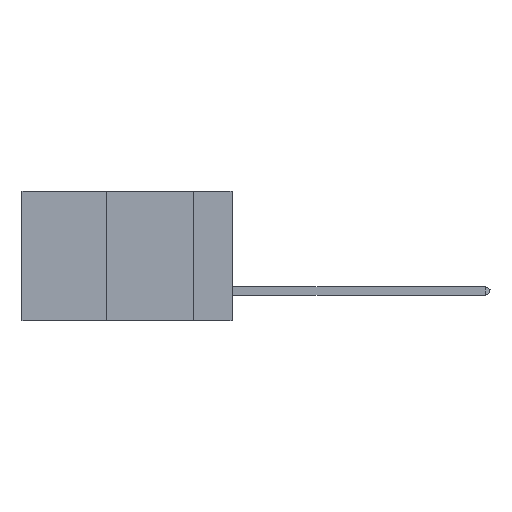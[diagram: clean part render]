
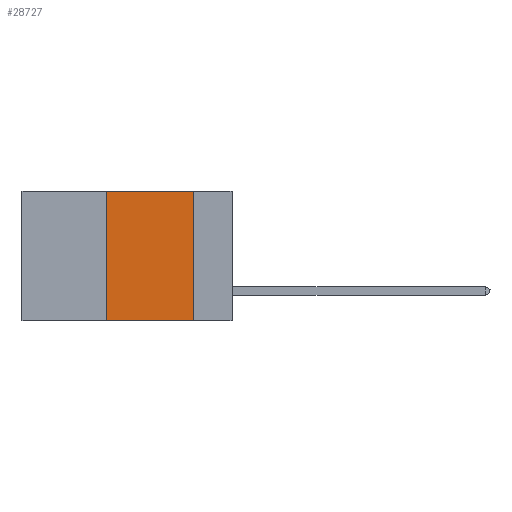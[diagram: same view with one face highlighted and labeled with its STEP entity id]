
A CAD part, left-side view. The second image highlights one B-rep face of the part: STEP entity #28727.
In plain terms, the highlighted planar face has unit normal (-1, 0, 0).
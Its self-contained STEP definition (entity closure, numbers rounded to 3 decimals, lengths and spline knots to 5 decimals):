
#2149 = DIRECTION ( 'NONE',  ( 0., -1., 0. ) ) ;
#2300 = CARTESIAN_POINT ( 'NONE',  ( 0., 0.6, 0. ) ) ;
#2467 = VERTEX_POINT ( 'NONE', #17054 ) ;
#5386 = CARTESIAN_POINT ( 'NONE',  ( 0., 0.36, -0.37 ) ) ;
#5473 = VECTOR ( 'NONE', #25019, 39.37008 ) ;
#6523 = EDGE_CURVE ( 'NONE', #19814, #19896, #8765, .T. ) ;
#8765 = LINE ( 'NONE', #23398, #31762 ) ;
#8870 = AXIS2_PLACEMENT_3D ( 'NONE', #43150, #19326, #15215 ) ;
#11661 = FACE_OUTER_BOUND ( 'NONE', #41821, .T. ) ;
#13138 = DIRECTION ( 'NONE',  ( 0., -1., 0. ) ) ;
#15215 = DIRECTION ( 'NONE',  ( 0., 0., -1. ) ) ;
#15361 = ORIENTED_EDGE ( 'NONE', *, *, #25147, .F. ) ;
#17054 = CARTESIAN_POINT ( 'NONE',  ( 0., 0.11, 0. ) ) ;
#17118 = LINE ( 'NONE', #45980, #36747 ) ;
#17146 = CARTESIAN_POINT ( 'NONE',  ( 0., 0.36, 0. ) ) ;
#19326 = DIRECTION ( 'NONE',  ( 1., 0., 0. ) ) ;
#19814 = VERTEX_POINT ( 'NONE', #5386 ) ;
#19896 = VERTEX_POINT ( 'NONE', #44915 ) ;
#20501 = ORIENTED_EDGE ( 'NONE', *, *, #31510, .F. ) ;
#21206 = DIRECTION ( 'NONE',  ( 0., 0., 1. ) ) ;
#23398 = CARTESIAN_POINT ( 'NONE',  ( 0., 0.6, -0.37 ) ) ;
#25019 = DIRECTION ( 'NONE',  ( 0., 0., -1. ) ) ;
#25147 = EDGE_CURVE ( 'NONE', #19814, #41192, #17118, .T. ) ;
#26268 = LINE ( 'NONE', #45852, #5473 ) ;
#28348 = LINE ( 'NONE', #2300, #32844 ) ;
#28727 = ADVANCED_FACE ( 'NONE', ( #11661 ), #39406, .F. ) ;
#31510 = EDGE_CURVE ( 'NONE', #41192, #2467, #28348, .T. ) ;
#31762 = VECTOR ( 'NONE', #2149, 39.37008 ) ;
#32844 = VECTOR ( 'NONE', #13138, 39.37008 ) ;
#36747 = VECTOR ( 'NONE', #21206, 39.37008 ) ;
#39386 = EDGE_CURVE ( 'NONE', #2467, #19896, #26268, .T. ) ;
#39406 = PLANE ( 'NONE',  #8870 ) ;
#41192 = VERTEX_POINT ( 'NONE', #17146 ) ;
#41821 = EDGE_LOOP ( 'NONE', ( #42415, #20501, #15361, #43810 ) ) ;
#42415 = ORIENTED_EDGE ( 'NONE', *, *, #39386, .F. ) ;
#43150 = CARTESIAN_POINT ( 'NONE',  ( 0., 0.6, 0. ) ) ;
#43810 = ORIENTED_EDGE ( 'NONE', *, *, #6523, .T. ) ;
#44915 = CARTESIAN_POINT ( 'NONE',  ( 0., 0.11, -0.37 ) ) ;
#45852 = CARTESIAN_POINT ( 'NONE',  ( 0., 0.11, 0. ) ) ;
#45980 = CARTESIAN_POINT ( 'NONE',  ( 0., 0.36, 0. ) ) ;
